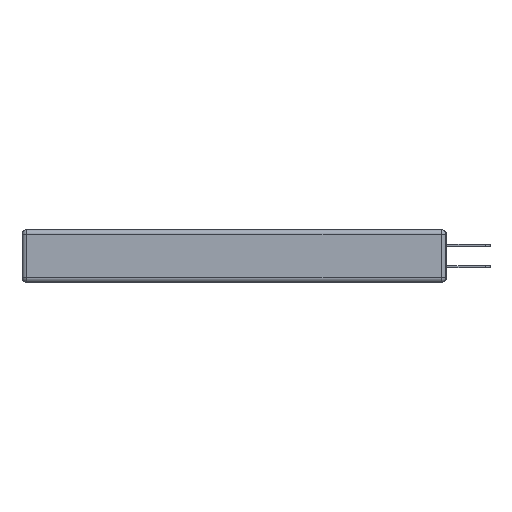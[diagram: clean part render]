
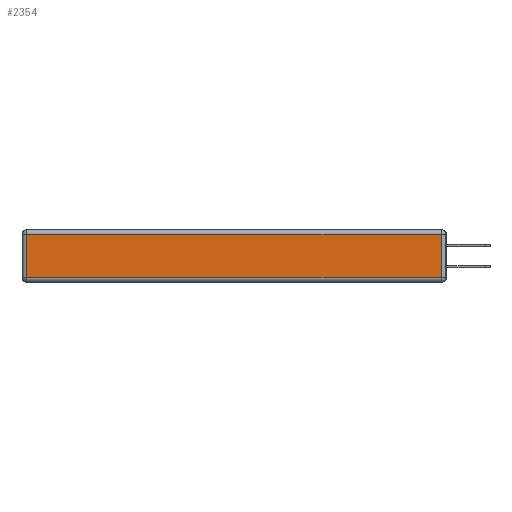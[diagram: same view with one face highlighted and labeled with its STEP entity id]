
A CAD part, left-side view. The second image highlights one B-rep face of the part: STEP entity #2354.
In plain terms, the highlighted planar face has unit normal (-1, 0, 0).
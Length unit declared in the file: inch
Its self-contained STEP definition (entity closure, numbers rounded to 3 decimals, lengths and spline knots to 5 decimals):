
#2193 = VERTEX_POINT ( 'NONE', #5321 ) ;
#2354 = ADVANCED_FACE ( 'NONE', ( #11810 ), #4009, .T. ) ;
#2458 = VERTEX_POINT ( 'NONE', #33582 ) ;
#2535 = DIRECTION ( 'NONE',  ( -1., 0., 0. ) ) ;
#4009 = PLANE ( 'NONE',  #8902 ) ;
#4251 = CARTESIAN_POINT ( 'NONE',  ( 0., 2.72, -0.03 ) ) ;
#5321 = CARTESIAN_POINT ( 'NONE',  ( 0., 0.03, -0.03 ) ) ;
#5757 = CARTESIAN_POINT ( 'NONE',  ( 0., 0., -0.343 ) ) ;
#5977 = VERTEX_POINT ( 'NONE', #14688 ) ;
#6079 = LINE ( 'NONE', #12061, #33052 ) ;
#6105 = LINE ( 'NONE', #28828, #7291 ) ;
#7291 = VECTOR ( 'NONE', #31213, 39.37008 ) ;
#8396 = VERTEX_POINT ( 'NONE', #4251 ) ;
#8535 = ORIENTED_EDGE ( 'NONE', *, *, #24090, .T. ) ;
#8902 = AXIS2_PLACEMENT_3D ( 'NONE', #5757, #2535, #30944 ) ;
#9045 = DIRECTION ( 'NONE',  ( 0., 1., 0. ) ) ;
#11298 = VECTOR ( 'NONE', #9045, 39.37008 ) ;
#11810 = FACE_OUTER_BOUND ( 'NONE', #25183, .T. ) ;
#12061 = CARTESIAN_POINT ( 'NONE',  ( 0., 0., -0.313 ) ) ;
#12907 = ORIENTED_EDGE ( 'NONE', *, *, #24346, .T. ) ;
#13546 = EDGE_CURVE ( 'NONE', #8396, #2458, #6105, .T. ) ;
#14688 = CARTESIAN_POINT ( 'NONE',  ( 0., 0.03, -0.313 ) ) ;
#16225 = ORIENTED_EDGE ( 'NONE', *, *, #20460, .T. ) ;
#16865 = CARTESIAN_POINT ( 'NONE',  ( 0., 2.75, -0.03 ) ) ;
#19109 = LINE ( 'NONE', #16865, #11298 ) ;
#20460 = EDGE_CURVE ( 'NONE', #5977, #2193, #21736, .T. ) ;
#21229 = ORIENTED_EDGE ( 'NONE', *, *, #13546, .T. ) ;
#21736 = LINE ( 'NONE', #29745, #28279 ) ;
#22616 = DIRECTION ( 'NONE',  ( 0., -1., 0. ) ) ;
#24090 = EDGE_CURVE ( 'NONE', #2193, #8396, #19109, .T. ) ;
#24346 = EDGE_CURVE ( 'NONE', #2458, #5977, #6079, .T. ) ;
#24933 = DIRECTION ( 'NONE',  ( 0., 0., 1. ) ) ;
#25183 = EDGE_LOOP ( 'NONE', ( #12907, #16225, #8535, #21229 ) ) ;
#28279 = VECTOR ( 'NONE', #24933, 39.37008 ) ;
#28828 = CARTESIAN_POINT ( 'NONE',  ( 0., 2.72, -0.343 ) ) ;
#29745 = CARTESIAN_POINT ( 'NONE',  ( 0., 0.03, -0.343 ) ) ;
#30944 = DIRECTION ( 'NONE',  ( 0., 0., 1. ) ) ;
#31213 = DIRECTION ( 'NONE',  ( 0., 0., -1. ) ) ;
#33052 = VECTOR ( 'NONE', #22616, 39.37008 ) ;
#33582 = CARTESIAN_POINT ( 'NONE',  ( 0., 2.72, -0.313 ) ) ;
